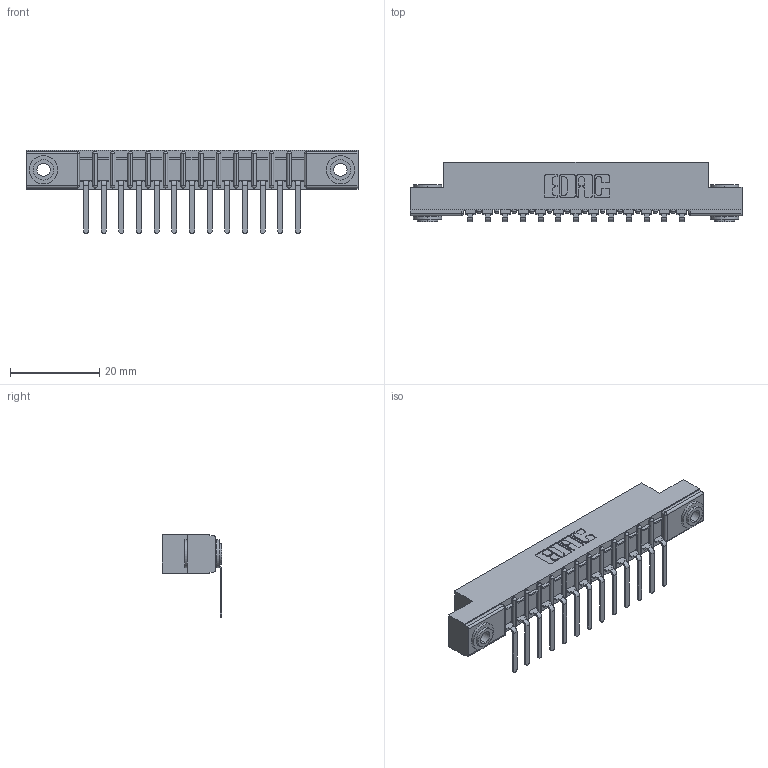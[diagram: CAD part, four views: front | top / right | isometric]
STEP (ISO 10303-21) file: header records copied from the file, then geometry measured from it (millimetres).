
FILE_DESCRIPTION (( 'STEP AP203' ), '1' );
FILE_NAME ('357-013-557-103.STEP', '2019-09-16T19:44:14', ( '' ), ( '' ), 'SwSTEP 2.0', 'SolidWorks 2016', '' );
FILE_SCHEMA (( 'CONFIG_CONTROL_DESIGN' ));
Length unit declared in the file: inch
Products named in the file (4): 307 Part_.156 Dia Mounting Holes; 345-250-002_345-250-002-102; 357-013-557-103; 307-290-002_557
Assembly tree (16 placements, depth 2):
  357-013-557-103
    307 Part_.156 Dia Mounting Holes
    307-290-002_557  x13
    345-250-002_345-250-002-102  x2
Bounding box: 74.52 x 13.36 x 18.67 mm (x, y, z)
Volume: 4951.6 mm3; surface area: 8964 mm2
Topology: 16 solids, 16 shells, 1198 faces, 3607 edges, 2362 vertices
Faces by surface type: plane 705, cylinder 457, sphere 28, cone 8
Entity records: 16639 total; most frequent: CARTESIAN_POINT 2781, ORIENTED_EDGE 2762, DIRECTION 2731, EDGE_CURVE 1381, LINE 1035, VECTOR 1035, VERTEX_POINT 898, AXIS2_PLACEMENT_3D 848
